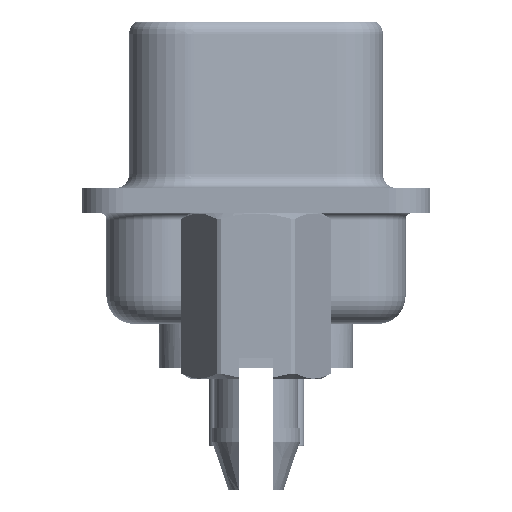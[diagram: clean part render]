
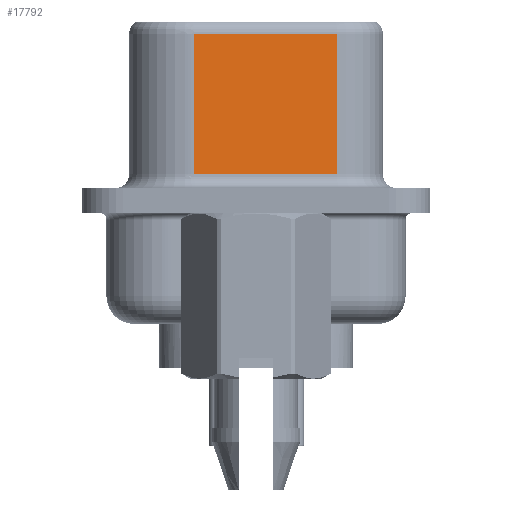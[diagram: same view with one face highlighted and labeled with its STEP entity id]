
A CAD part, left-side view. The second image highlights one B-rep face of the part: STEP entity #17792.
In plain terms, the highlighted planar face has unit normal (-0.985, -0.174, 0).
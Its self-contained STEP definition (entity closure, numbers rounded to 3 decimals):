
#1733 = EDGE_CURVE ( 'NONE', #19569, #16747, #3243, .T. ) ;
#2093 = CARTESIAN_POINT ( 'NONE',  ( 4.58, -2.927, 0.95 ) ) ;
#3243 = LINE ( 'NONE', #8267, #6572 ) ;
#3408 = DIRECTION ( 'NONE',  ( 0., 0., -1. ) ) ;
#4997 = VERTEX_POINT ( 'NONE', #5068 ) ;
#5068 = CARTESIAN_POINT ( 'NONE',  ( 3.67, 2.233, 6.02 ) ) ;
#5589 = CARTESIAN_POINT ( 'NONE',  ( 3.67, 2.233, 0.95 ) ) ;
#6572 = VECTOR ( 'NONE', #3408, 1000. ) ;
#8267 = CARTESIAN_POINT ( 'NONE',  ( 4.58, -2.927, 6.52 ) ) ;
#8629 = PLANE ( 'NONE',  #10552 ) ;
#8637 = EDGE_CURVE ( 'NONE', #11182, #16747, #18088, .T. ) ;
#9986 = VECTOR ( 'NONE', #18795, 1000. ) ;
#10552 = AXIS2_PLACEMENT_3D ( 'NONE', #27580, #13376, #29963 ) ;
#10624 = DIRECTION ( 'NONE',  ( 0.174, -0.985, 0. ) ) ;
#11182 = VERTEX_POINT ( 'NONE', #5589 ) ;
#11221 = EDGE_LOOP ( 'NONE', ( #26572, #26174, #18781, #16159 ) ) ;
#11786 = VECTOR ( 'NONE', #10624, 1000. ) ;
#12988 = CARTESIAN_POINT ( 'NONE',  ( 4.58, -2.927, 0.95 ) ) ;
#13059 = DIRECTION ( 'NONE',  ( 0., 0., -1. ) ) ;
#13376 = DIRECTION ( 'NONE',  ( 0.985, 0.174, 0. ) ) ;
#16159 = ORIENTED_EDGE ( 'NONE', *, *, #8637, .T. ) ;
#16747 = VERTEX_POINT ( 'NONE', #2093 ) ;
#17792 = ADVANCED_FACE ( 'NONE', ( #22216 ), #8629, .F. ) ;
#18088 = LINE ( 'NONE', #12988, #11786 ) ;
#18781 = ORIENTED_EDGE ( 'NONE', *, *, #20382, .T. ) ;
#18795 = DIRECTION ( 'NONE',  ( -0.174, 0.985, 0. ) ) ;
#19569 = VERTEX_POINT ( 'NONE', #21910 ) ;
#19862 = VECTOR ( 'NONE', #13059, 1000. ) ;
#20382 = EDGE_CURVE ( 'NONE', #4997, #11182, #26124, .T. ) ;
#21910 = CARTESIAN_POINT ( 'NONE',  ( 4.58, -2.927, 6.02 ) ) ;
#22216 = FACE_OUTER_BOUND ( 'NONE', #11221, .T. ) ;
#23326 = LINE ( 'NONE', #30617, #9986 ) ;
#24392 = EDGE_CURVE ( 'NONE', #19569, #4997, #23326, .T. ) ;
#26124 = LINE ( 'NONE', #29751, #19862 ) ;
#26174 = ORIENTED_EDGE ( 'NONE', *, *, #24392, .T. ) ;
#26572 = ORIENTED_EDGE ( 'NONE', *, *, #1733, .F. ) ;
#27580 = CARTESIAN_POINT ( 'NONE',  ( 4.58, -2.927, 6.52 ) ) ;
#29751 = CARTESIAN_POINT ( 'NONE',  ( 3.67, 2.233, 6.52 ) ) ;
#29963 = DIRECTION ( 'NONE',  ( -0.174, 0.985, 0. ) ) ;
#30617 = CARTESIAN_POINT ( 'NONE',  ( 4.58, -2.927, 6.02 ) ) ;
